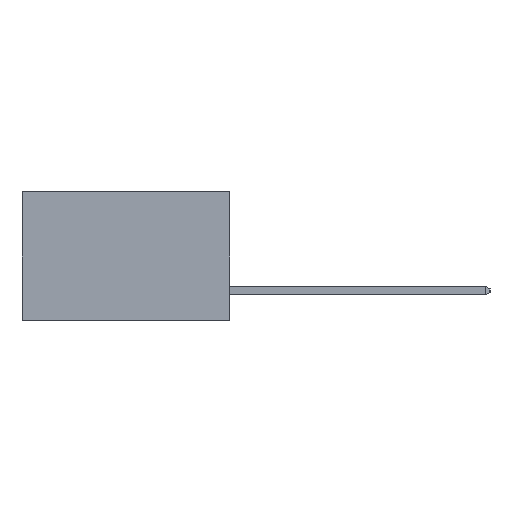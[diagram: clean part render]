
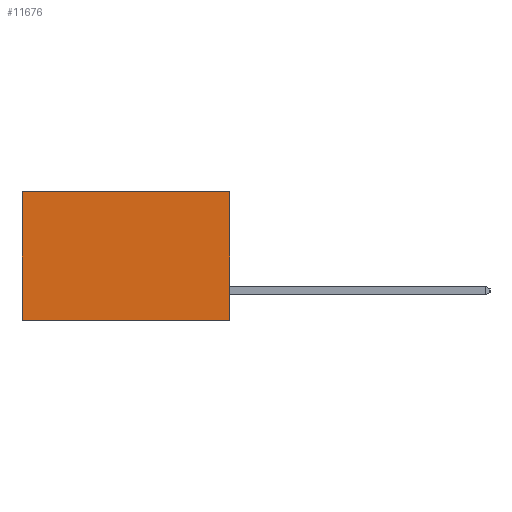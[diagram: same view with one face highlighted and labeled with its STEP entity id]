
A CAD part, left-side view. The second image highlights one B-rep face of the part: STEP entity #11676.
In plain terms, the highlighted planar face has unit normal (-1, 0, 0).
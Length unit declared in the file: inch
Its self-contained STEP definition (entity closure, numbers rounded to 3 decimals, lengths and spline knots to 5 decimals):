
#52 = FACE_OUTER_BOUND ( 'NONE', #14367, .T. ) ;
#185 = EDGE_CURVE ( 'NONE', #12785, #15130, #11523, .T. ) ;
#990 = VECTOR ( 'NONE', #15030, 39.37008 ) ;
#1431 = LINE ( 'NONE', #9810, #990 ) ;
#2328 = CARTESIAN_POINT ( 'NONE',  ( 0.2615, 0., 0. ) ) ;
#3686 = CARTESIAN_POINT ( 'NONE',  ( 0.2615, 0.6, -0.37 ) ) ;
#3941 = VECTOR ( 'NONE', #9240, 39.37008 ) ;
#4546 = ORIENTED_EDGE ( 'NONE', *, *, #12697, .T. ) ;
#5072 = CARTESIAN_POINT ( 'NONE',  ( 0.2615, 0., 0. ) ) ;
#6336 = VERTEX_POINT ( 'NONE', #9257 ) ;
#6515 = CARTESIAN_POINT ( 'NONE',  ( 0.2615, 0., -0.37 ) ) ;
#9093 = DIRECTION ( 'NONE',  ( 0., 1., 0. ) ) ;
#9240 = DIRECTION ( 'NONE',  ( 0., 1., 0. ) ) ;
#9257 = CARTESIAN_POINT ( 'NONE',  ( 0.2615, 0.6, 0. ) ) ;
#9354 = EDGE_CURVE ( 'NONE', #6336, #15130, #14074, .T. ) ;
#9810 = CARTESIAN_POINT ( 'NONE',  ( 0.2615, 0., -0.37 ) ) ;
#10327 = ORIENTED_EDGE ( 'NONE', *, *, #9354, .T. ) ;
#11052 = DIRECTION ( 'NONE',  ( 0., 0., -1. ) ) ;
#11070 = DIRECTION ( 'NONE',  ( 1., 0., 0. ) ) ;
#11217 = CARTESIAN_POINT ( 'NONE',  ( 0.2615, 0., -0.37 ) ) ;
#11431 = ORIENTED_EDGE ( 'NONE', *, *, #185, .F. ) ;
#11523 = LINE ( 'NONE', #14952, #3941 ) ;
#11534 = PLANE ( 'NONE',  #12751 ) ;
#11676 = ADVANCED_FACE ( 'NONE', ( #52 ), #11534, .F. ) ;
#12697 = EDGE_CURVE ( 'NONE', #15993, #6336, #16297, .T. ) ;
#12751 = AXIS2_PLACEMENT_3D ( 'NONE', #11217, #11070, #11052 ) ;
#12785 = VERTEX_POINT ( 'NONE', #6515 ) ;
#13270 = VECTOR ( 'NONE', #15758, 39.37008 ) ;
#14074 = LINE ( 'NONE', #15811, #13270 ) ;
#14367 = EDGE_LOOP ( 'NONE', ( #10327, #11431, #15391, #4546 ) ) ;
#14952 = CARTESIAN_POINT ( 'NONE',  ( 0.2615, 0., -0.37 ) ) ;
#15030 = DIRECTION ( 'NONE',  ( 0., 0., -1. ) ) ;
#15130 = VERTEX_POINT ( 'NONE', #3686 ) ;
#15391 = ORIENTED_EDGE ( 'NONE', *, *, #15687, .F. ) ;
#15687 = EDGE_CURVE ( 'NONE', #15993, #12785, #1431, .T. ) ;
#15758 = DIRECTION ( 'NONE',  ( 0., 0., -1. ) ) ;
#15811 = CARTESIAN_POINT ( 'NONE',  ( 0.2615, 0.6, -0.37 ) ) ;
#15907 = VECTOR ( 'NONE', #9093, 39.37008 ) ;
#15993 = VERTEX_POINT ( 'NONE', #5072 ) ;
#16297 = LINE ( 'NONE', #2328, #15907 ) ;
